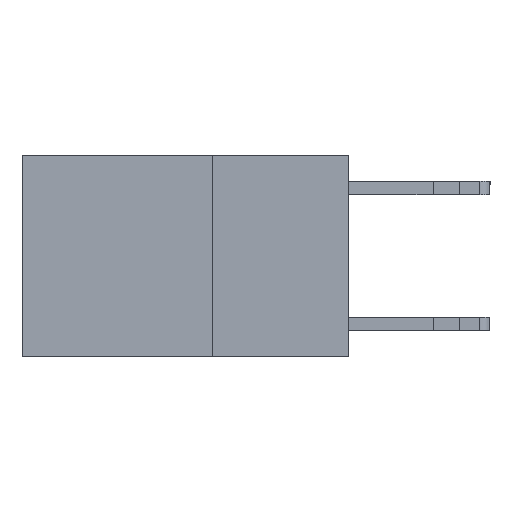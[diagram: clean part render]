
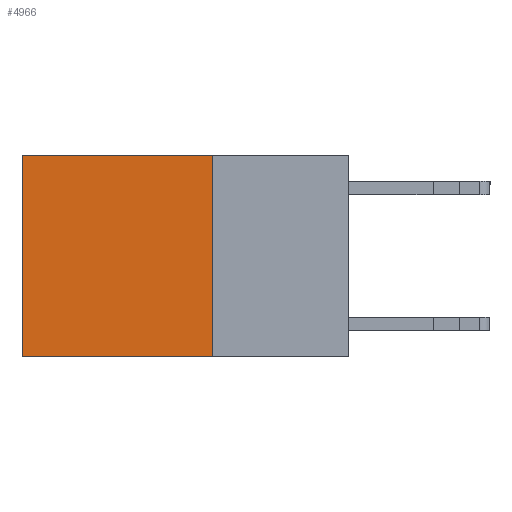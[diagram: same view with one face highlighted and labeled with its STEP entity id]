
A CAD part, left-side view. The second image highlights one B-rep face of the part: STEP entity #4966.
In plain terms, the highlighted planar face has unit normal (-1, 0, 0).
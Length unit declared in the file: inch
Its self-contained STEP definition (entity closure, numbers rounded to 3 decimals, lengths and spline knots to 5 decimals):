
#885 = CARTESIAN_POINT ( 'NONE',  ( 0.2625, 0.25, 0. ) ) ;
#929 = DIRECTION ( 'NONE',  ( 1., 0., 0. ) ) ;
#1046 = VECTOR ( 'NONE', #6698, 39.37008 ) ;
#1047 = CARTESIAN_POINT ( 'NONE',  ( 0.2625, 0.25, 0. ) ) ;
#1163 = VECTOR ( 'NONE', #1464, 39.37008 ) ;
#1464 = DIRECTION ( 'NONE',  ( 0., 1., 0. ) ) ;
#1526 = CARTESIAN_POINT ( 'NONE',  ( 0.2625, 0.25, -0.37 ) ) ;
#1680 = LINE ( 'NONE', #6953, #9320 ) ;
#2122 = EDGE_CURVE ( 'NONE', #11535, #4520, #1680, .T. ) ;
#2398 = DIRECTION ( 'NONE',  ( 0., 0., -1. ) ) ;
#2413 = ORIENTED_EDGE ( 'NONE', *, *, #7329, .F. ) ;
#2590 = CARTESIAN_POINT ( 'NONE',  ( 0.2625, 0.25, -0.37 ) ) ;
#3434 = LINE ( 'NONE', #1526, #1163 ) ;
#4510 = DIRECTION ( 'NONE',  ( 0., 0., -1. ) ) ;
#4520 = VERTEX_POINT ( 'NONE', #9313 ) ;
#4642 = DIRECTION ( 'NONE',  ( 0., 0., -1. ) ) ;
#4814 = ORIENTED_EDGE ( 'NONE', *, *, #9615, .T. ) ;
#4966 = ADVANCED_FACE ( 'NONE', ( #10128 ), #7525, .F. ) ;
#5242 = EDGE_CURVE ( 'NONE', #5755, #4520, #3434, .T. ) ;
#5755 = VERTEX_POINT ( 'NONE', #2590 ) ;
#5823 = CARTESIAN_POINT ( 'NONE',  ( 0.2625, 0.6, 0. ) ) ;
#5968 = VECTOR ( 'NONE', #4642, 39.37008 ) ;
#6445 = LINE ( 'NONE', #9018, #5968 ) ;
#6698 = DIRECTION ( 'NONE',  ( 0., 1., 0. ) ) ;
#6953 = CARTESIAN_POINT ( 'NONE',  ( 0.2625, 0.6, 0. ) ) ;
#7287 = EDGE_LOOP ( 'NONE', ( #10164, #11257, #2413, #4814 ) ) ;
#7291 = AXIS2_PLACEMENT_3D ( 'NONE', #1047, #929, #4510 ) ;
#7329 = EDGE_CURVE ( 'NONE', #9349, #5755, #6445, .T. ) ;
#7525 = PLANE ( 'NONE',  #7291 ) ;
#9018 = CARTESIAN_POINT ( 'NONE',  ( 0.2625, 0.25, 0. ) ) ;
#9082 = LINE ( 'NONE', #885, #1046 ) ;
#9313 = CARTESIAN_POINT ( 'NONE',  ( 0.2625, 0.6, -0.37 ) ) ;
#9320 = VECTOR ( 'NONE', #2398, 39.37008 ) ;
#9349 = VERTEX_POINT ( 'NONE', #10749 ) ;
#9615 = EDGE_CURVE ( 'NONE', #9349, #11535, #9082, .T. ) ;
#10128 = FACE_OUTER_BOUND ( 'NONE', #7287, .T. ) ;
#10164 = ORIENTED_EDGE ( 'NONE', *, *, #2122, .T. ) ;
#10749 = CARTESIAN_POINT ( 'NONE',  ( 0.2625, 0.25, 0. ) ) ;
#11257 = ORIENTED_EDGE ( 'NONE', *, *, #5242, .F. ) ;
#11535 = VERTEX_POINT ( 'NONE', #5823 ) ;
